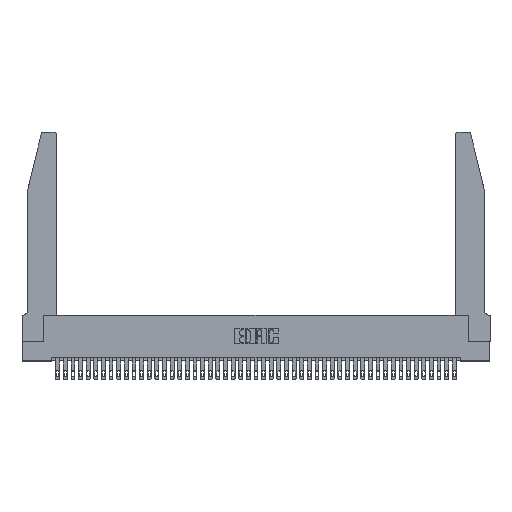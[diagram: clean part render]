
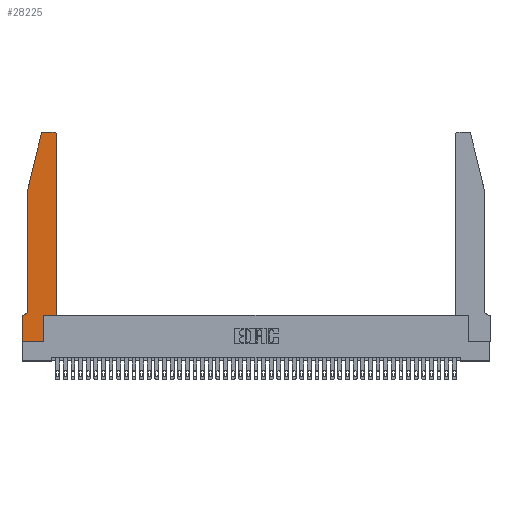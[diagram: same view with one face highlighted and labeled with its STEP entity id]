
A CAD part, top view. The second image highlights one B-rep face of the part: STEP entity #28225.
In plain terms, the highlighted planar face has unit normal (0, 0, 1).
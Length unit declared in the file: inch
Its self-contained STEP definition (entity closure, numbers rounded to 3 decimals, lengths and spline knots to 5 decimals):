
#237 = ORIENTED_EDGE ( 'NONE', *, *, #16773, .T. ) ;
#326 = CIRCLE ( 'NONE', #29587, 0.03 ) ;
#785 = ORIENTED_EDGE ( 'NONE', *, *, #11540, .T. ) ;
#1130 = DIRECTION ( 'NONE',  ( -1., 0., 0. ) ) ;
#1322 = LINE ( 'NONE', #17376, #37145 ) ;
#1464 = VECTOR ( 'NONE', #35307, 39.37008 ) ;
#2831 = CARTESIAN_POINT ( 'NONE',  ( 0., 0., 0.37 ) ) ;
#3650 = CARTESIAN_POINT ( 'NONE',  ( 0., 0.35, 0.37 ) ) ;
#4043 = CARTESIAN_POINT ( 'NONE',  ( 0.4505, 2.72, 0.37 ) ) ;
#4227 = CARTESIAN_POINT ( 'NONE',  ( 0.2865, 0.35, 0.37 ) ) ;
#4278 = CARTESIAN_POINT ( 'NONE',  ( 0., 0.35, 0.37 ) ) ;
#4481 = DIRECTION ( 'NONE',  ( 0., -1., 0. ) ) ;
#5019 = CARTESIAN_POINT ( 'NONE',  ( 0.0755, 0.42, 0.37 ) ) ;
#8238 = ORIENTED_EDGE ( 'NONE', *, *, #38332, .T. ) ;
#8360 = ORIENTED_EDGE ( 'NONE', *, *, #19345, .T. ) ;
#8958 = CARTESIAN_POINT ( 'NONE',  ( 0., 0., 0.37 ) ) ;
#10014 = LINE ( 'NONE', #20930, #25189 ) ;
#10284 = ORIENTED_EDGE ( 'NONE', *, *, #16746, .T. ) ;
#10434 = CARTESIAN_POINT ( 'NONE',  ( 0.2865, 0.35, 0.37 ) ) ;
#10807 = EDGE_LOOP ( 'NONE', ( #43767, #8360, #25740, #21420, #33263, #237, #42383, #41537, #785, #23719, #8238, #10284 ) ) ;
#10964 = CARTESIAN_POINT ( 'NONE',  ( 0.0055, 0.42, 0.37 ) ) ;
#11540 = EDGE_CURVE ( 'NONE', #14436, #33036, #16208, .T. ) ;
#11798 = LINE ( 'NONE', #32079, #43757 ) ;
#12334 = DIRECTION ( 'NONE',  ( -0.239, -0.971, 0. ) ) ;
#12507 = CIRCLE ( 'NONE', #20443, 0.03 ) ;
#13562 = LINE ( 'NONE', #20202, #28193 ) ;
#13666 = CIRCLE ( 'NONE', #36188, 0.07 ) ;
#14069 = AXIS2_PLACEMENT_3D ( 'NONE', #3650, #27930, #17626 ) ;
#14316 = EDGE_CURVE ( 'NONE', #21352, #16691, #1322, .T. ) ;
#14436 = VERTEX_POINT ( 'NONE', #32543 ) ;
#14659 = VECTOR ( 'NONE', #1130, 39.37008 ) ;
#15441 = VERTEX_POINT ( 'NONE', #25297 ) ;
#15952 = DIRECTION ( 'NONE',  ( 1., 0., 0. ) ) ;
#16208 = LINE ( 'NONE', #4227, #1464 ) ;
#16414 = CARTESIAN_POINT ( 'NONE',  ( 0.4205, 2.72, 0.37 ) ) ;
#16691 = VERTEX_POINT ( 'NONE', #33957 ) ;
#16746 = EDGE_CURVE ( 'NONE', #44232, #21352, #12507, .T. ) ;
#16773 = EDGE_CURVE ( 'NONE', #15441, #21082, #32560, .T. ) ;
#17376 = CARTESIAN_POINT ( 'NONE',  ( 0.2605, 2.75, 0.37 ) ) ;
#17626 = DIRECTION ( 'NONE',  ( 1., 0., 0. ) ) ;
#17812 = LINE ( 'NONE', #33137, #38382 ) ;
#18262 = DIRECTION ( 'NONE',  ( 0., 0., -1. ) ) ;
#18848 = EDGE_CURVE ( 'NONE', #28206, #36887, #11798, .T. ) ;
#18929 = CARTESIAN_POINT ( 'NONE',  ( 0., 0., 0.37 ) ) ;
#19345 = EDGE_CURVE ( 'NONE', #16691, #24232, #326, .T. ) ;
#20202 = CARTESIAN_POINT ( 'NONE',  ( 0.4505, 0.35, 0.37 ) ) ;
#20443 = AXIS2_PLACEMENT_3D ( 'NONE', #16414, #44345, #40573 ) ;
#20744 = EDGE_CURVE ( 'NONE', #29292, #14436, #42444, .T. ) ;
#20930 = CARTESIAN_POINT ( 'NONE',  ( 0.4505, 0.35, 0.37 ) ) ;
#20966 = CARTESIAN_POINT ( 'NONE',  ( 0.4505, 0.35, 0.37 ) ) ;
#21040 = FACE_OUTER_BOUND ( 'NONE', #10807, .T. ) ;
#21082 = VERTEX_POINT ( 'NONE', #4278 ) ;
#21352 = VERTEX_POINT ( 'NONE', #31312 ) ;
#21420 = ORIENTED_EDGE ( 'NONE', *, *, #18848, .T. ) ;
#21807 = CARTESIAN_POINT ( 'NONE',  ( 0.25487, 2.72718, 0.37 ) ) ;
#23719 = ORIENTED_EDGE ( 'NONE', *, *, #30968, .T. ) ;
#24232 = VERTEX_POINT ( 'NONE', #21807 ) ;
#24447 = DIRECTION ( 'NONE',  ( 1., 0., 0. ) ) ;
#24469 = PLANE ( 'NONE',  #14069 ) ;
#25189 = VECTOR ( 'NONE', #24447, 39.37008 ) ;
#25297 = CARTESIAN_POINT ( 'NONE',  ( 0.0055, 0.35, 0.37 ) ) ;
#25740 = ORIENTED_EDGE ( 'NONE', *, *, #27949, .T. ) ;
#26683 = EDGE_CURVE ( 'NONE', #21082, #29292, #42748, .T. ) ;
#27616 = DIRECTION ( 'NONE',  ( 0., 1., 0. ) ) ;
#27930 = DIRECTION ( 'NONE',  ( 0., 0., 1. ) ) ;
#27949 = EDGE_CURVE ( 'NONE', #24232, #28206, #17812, .T. ) ;
#28193 = VECTOR ( 'NONE', #27616, 39.37008 ) ;
#28206 = VERTEX_POINT ( 'NONE', #38192 ) ;
#28225 = ADVANCED_FACE ( 'NONE', ( #21040 ), #24469, .T. ) ;
#29292 = VERTEX_POINT ( 'NONE', #2831 ) ;
#29492 = DIRECTION ( 'NONE',  ( 1., 0., 0. ) ) ;
#29587 = AXIS2_PLACEMENT_3D ( 'NONE', #30275, #41405, #15952 ) ;
#30275 = CARTESIAN_POINT ( 'NONE',  ( 0.284, 2.72, 0.37 ) ) ;
#30968 = EDGE_CURVE ( 'NONE', #33036, #43558, #10014, .T. ) ;
#31312 = CARTESIAN_POINT ( 'NONE',  ( 0.4205, 2.75, 0.37 ) ) ;
#32079 = CARTESIAN_POINT ( 'NONE',  ( 0.0755, 2., 0.37 ) ) ;
#32543 = CARTESIAN_POINT ( 'NONE',  ( 0.2865, 0., 0.37 ) ) ;
#32560 = LINE ( 'NONE', #34263, #14659 ) ;
#33036 = VERTEX_POINT ( 'NONE', #10434 ) ;
#33137 = CARTESIAN_POINT ( 'NONE',  ( 0.0755, 2., 0.37 ) ) ;
#33263 = ORIENTED_EDGE ( 'NONE', *, *, #42840, .T. ) ;
#33650 = VECTOR ( 'NONE', #43093, 39.37008 ) ;
#33957 = CARTESIAN_POINT ( 'NONE',  ( 0.284, 2.75, 0.37 ) ) ;
#34263 = CARTESIAN_POINT ( 'NONE',  ( 0.0755, 0.35, 0.37 ) ) ;
#35307 = DIRECTION ( 'NONE',  ( 0., 1., 0. ) ) ;
#36188 = AXIS2_PLACEMENT_3D ( 'NONE', #10964, #18262, #38541 ) ;
#36887 = VERTEX_POINT ( 'NONE', #5019 ) ;
#37145 = VECTOR ( 'NONE', #42249, 39.37008 ) ;
#38192 = CARTESIAN_POINT ( 'NONE',  ( 0.0755, 2., 0.37 ) ) ;
#38332 = EDGE_CURVE ( 'NONE', #43558, #44232, #13562, .T. ) ;
#38382 = VECTOR ( 'NONE', #12334, 39.37008 ) ;
#38541 = DIRECTION ( 'NONE',  ( -1., 0., 0. ) ) ;
#39206 = VECTOR ( 'NONE', #29492, 39.37008 ) ;
#40573 = DIRECTION ( 'NONE',  ( 1., 0., 0. ) ) ;
#41405 = DIRECTION ( 'NONE',  ( 0., 0., 1. ) ) ;
#41537 = ORIENTED_EDGE ( 'NONE', *, *, #20744, .T. ) ;
#42249 = DIRECTION ( 'NONE',  ( -1., 0., 0. ) ) ;
#42383 = ORIENTED_EDGE ( 'NONE', *, *, #26683, .T. ) ;
#42444 = LINE ( 'NONE', #8958, #39206 ) ;
#42748 = LINE ( 'NONE', #18929, #33650 ) ;
#42840 = EDGE_CURVE ( 'NONE', #36887, #15441, #13666, .T. ) ;
#43093 = DIRECTION ( 'NONE',  ( 0., -1., 0. ) ) ;
#43558 = VERTEX_POINT ( 'NONE', #20966 ) ;
#43757 = VECTOR ( 'NONE', #4481, 39.37008 ) ;
#43767 = ORIENTED_EDGE ( 'NONE', *, *, #14316, .T. ) ;
#44232 = VERTEX_POINT ( 'NONE', #4043 ) ;
#44345 = DIRECTION ( 'NONE',  ( 0., 0., 1. ) ) ;
